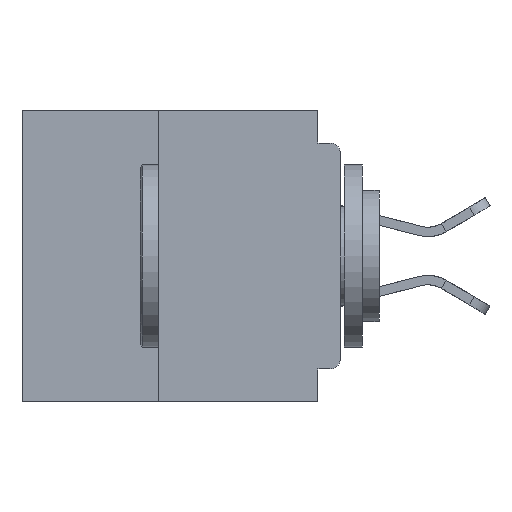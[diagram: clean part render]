
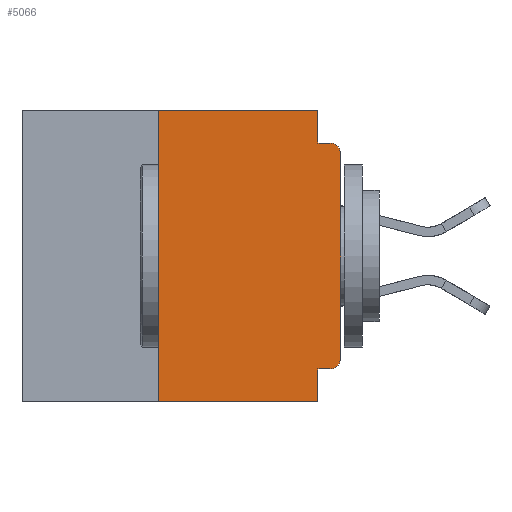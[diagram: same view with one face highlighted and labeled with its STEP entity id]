
A CAD part, left-side view. The second image highlights one B-rep face of the part: STEP entity #5066.
In plain terms, the highlighted planar face has unit normal (-1, 0, 0).
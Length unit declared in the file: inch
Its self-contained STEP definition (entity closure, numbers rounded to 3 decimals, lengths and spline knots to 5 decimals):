
#410 = VERTEX_POINT ( 'NONE', #44594 ) ;
#521 = CARTESIAN_POINT ( 'NONE',  ( 0., 0.015, -0.045 ) ) ;
#858 = CARTESIAN_POINT ( 'NONE',  ( 0., 0.25, -0.4 ) ) ;
#1553 = VERTEX_POINT ( 'NONE', #38633 ) ;
#1782 = EDGE_CURVE ( 'NONE', #38495, #410, #31186, .T. ) ;
#2351 = VECTOR ( 'NONE', #15115, 39.37008 ) ;
#2482 = LINE ( 'NONE', #26480, #40774 ) ;
#2640 = DIRECTION ( 'NONE',  ( 0., 0., -1. ) ) ;
#2669 = DIRECTION ( 'NONE',  ( 0., 0., -1. ) ) ;
#3122 = DIRECTION ( 'NONE',  ( 0., -1., 0. ) ) ;
#3851 = EDGE_CURVE ( 'NONE', #36804, #38495, #11431, .T. ) ;
#5031 = VECTOR ( 'NONE', #39008, 39.37008 ) ;
#5066 = ADVANCED_FACE ( 'NONE', ( #44880 ), #32193, .F. ) ;
#5093 = EDGE_CURVE ( 'NONE', #30592, #1553, #25356, .T. ) ;
#5676 = AXIS2_PLACEMENT_3D ( 'NONE', #14829, #40547, #18569 ) ;
#6578 = ORIENTED_EDGE ( 'NONE', *, *, #15132, .T. ) ;
#6948 = EDGE_CURVE ( 'NONE', #1553, #24977, #2482, .T. ) ;
#7281 = VERTEX_POINT ( 'NONE', #17346 ) ;
#7974 = CARTESIAN_POINT ( 'NONE',  ( 0., 0.031, 0. ) ) ;
#8047 = EDGE_CURVE ( 'NONE', #7281, #14858, #14187, .T. ) ;
#8215 = ORIENTED_EDGE ( 'NONE', *, *, #16314, .F. ) ;
#8944 = CARTESIAN_POINT ( 'NONE',  ( 0., 0.031, -0.355 ) ) ;
#9020 = DIRECTION ( 'NONE',  ( 0., 0., -1. ) ) ;
#9783 = AXIS2_PLACEMENT_3D ( 'NONE', #21483, #47158, #25150 ) ;
#10757 = CARTESIAN_POINT ( 'NONE',  ( 0., 0.031, 0. ) ) ;
#11431 = LINE ( 'NONE', #32276, #20201 ) ;
#12268 = DIRECTION ( 'NONE',  ( 0., 0., 1. ) ) ;
#12294 = AXIS2_PLACEMENT_3D ( 'NONE', #46854, #24986, #2640 ) ;
#12662 = LINE ( 'NONE', #28679, #29947 ) ;
#14187 = LINE ( 'NONE', #18089, #21715 ) ;
#14800 = VERTEX_POINT ( 'NONE', #8944 ) ;
#14829 = CARTESIAN_POINT ( 'NONE',  ( 0., 0.015, -0.06 ) ) ;
#14858 = VERTEX_POINT ( 'NONE', #31234 ) ;
#15036 = LINE ( 'NONE', #42671, #5031 ) ;
#15115 = DIRECTION ( 'NONE',  ( 0., -1., 0. ) ) ;
#15132 = EDGE_CURVE ( 'NONE', #24977, #17770, #23715, .T. ) ;
#16197 = EDGE_CURVE ( 'NONE', #30592, #14800, #15036, .T. ) ;
#16314 = EDGE_CURVE ( 'NONE', #14800, #14858, #12662, .T. ) ;
#17346 = CARTESIAN_POINT ( 'NONE',  ( 0., 0.25, -0.4 ) ) ;
#17770 = VERTEX_POINT ( 'NONE', #521 ) ;
#18029 = EDGE_LOOP ( 'NONE', ( #35702, #6578, #40724, #28450, #26901, #32631, #36878, #8215, #34798, #23837 ) ) ;
#18089 = CARTESIAN_POINT ( 'NONE',  ( 0., 0.437, -0.4 ) ) ;
#18569 = DIRECTION ( 'NONE',  ( 0., 0., -1. ) ) ;
#20201 = VECTOR ( 'NONE', #46948, 39.37008 ) ;
#21483 = CARTESIAN_POINT ( 'NONE',  ( 0., 0.015, -0.34 ) ) ;
#21715 = VECTOR ( 'NONE', #3122, 39.37008 ) ;
#23715 = CIRCLE ( 'NONE', #5676, 0.015 ) ;
#23837 = ORIENTED_EDGE ( 'NONE', *, *, #5093, .T. ) ;
#24977 = VERTEX_POINT ( 'NONE', #38444 ) ;
#24986 = DIRECTION ( 'NONE',  ( 1., 0., 0. ) ) ;
#25150 = DIRECTION ( 'NONE',  ( 0., 0., -1. ) ) ;
#25345 = EDGE_CURVE ( 'NONE', #410, #17770, #28521, .T. ) ;
#25356 = CIRCLE ( 'NONE', #9783, 0.015 ) ;
#25401 = VECTOR ( 'NONE', #12268, 39.37008 ) ;
#25553 = CARTESIAN_POINT ( 'NONE',  ( 0., 0.015, -0.355 ) ) ;
#26480 = CARTESIAN_POINT ( 'NONE',  ( 0., 0., 0. ) ) ;
#26901 = ORIENTED_EDGE ( 'NONE', *, *, #3851, .F. ) ;
#28450 = ORIENTED_EDGE ( 'NONE', *, *, #1782, .F. ) ;
#28521 = LINE ( 'NONE', #37136, #2351 ) ;
#28679 = CARTESIAN_POINT ( 'NONE',  ( 0., 0.031, -0.4 ) ) ;
#29947 = VECTOR ( 'NONE', #2669, 39.37008 ) ;
#30592 = VERTEX_POINT ( 'NONE', #25553 ) ;
#31186 = LINE ( 'NONE', #10757, #39849 ) ;
#31234 = CARTESIAN_POINT ( 'NONE',  ( 0., 0.031, -0.4 ) ) ;
#32193 = PLANE ( 'NONE',  #12294 ) ;
#32276 = CARTESIAN_POINT ( 'NONE',  ( 0., 0.437, 0. ) ) ;
#32631 = ORIENTED_EDGE ( 'NONE', *, *, #37992, .F. ) ;
#34472 = CARTESIAN_POINT ( 'NONE',  ( 0., 0.25, 0. ) ) ;
#34798 = ORIENTED_EDGE ( 'NONE', *, *, #16197, .F. ) ;
#35155 = LINE ( 'NONE', #858, #25401 ) ;
#35702 = ORIENTED_EDGE ( 'NONE', *, *, #6948, .T. ) ;
#36804 = VERTEX_POINT ( 'NONE', #34472 ) ;
#36878 = ORIENTED_EDGE ( 'NONE', *, *, #8047, .T. ) ;
#37136 = CARTESIAN_POINT ( 'NONE',  ( 0., 0., -0.045 ) ) ;
#37582 = DIRECTION ( 'NONE',  ( 0., 0., 1. ) ) ;
#37992 = EDGE_CURVE ( 'NONE', #7281, #36804, #35155, .T. ) ;
#38444 = CARTESIAN_POINT ( 'NONE',  ( 0., 0., -0.06 ) ) ;
#38495 = VERTEX_POINT ( 'NONE', #7974 ) ;
#38633 = CARTESIAN_POINT ( 'NONE',  ( 0., 0., -0.34 ) ) ;
#39008 = DIRECTION ( 'NONE',  ( 0., 1., 0. ) ) ;
#39849 = VECTOR ( 'NONE', #9020, 39.37008 ) ;
#40547 = DIRECTION ( 'NONE',  ( -1., 0., 0. ) ) ;
#40724 = ORIENTED_EDGE ( 'NONE', *, *, #25345, .F. ) ;
#40774 = VECTOR ( 'NONE', #37582, 39.37008 ) ;
#42671 = CARTESIAN_POINT ( 'NONE',  ( 0., 0., -0.355 ) ) ;
#44594 = CARTESIAN_POINT ( 'NONE',  ( 0., 0.031, -0.045 ) ) ;
#44880 = FACE_OUTER_BOUND ( 'NONE', #18029, .T. ) ;
#46854 = CARTESIAN_POINT ( 'NONE',  ( 0., 0.437, 0. ) ) ;
#46948 = DIRECTION ( 'NONE',  ( 0., -1., 0. ) ) ;
#47158 = DIRECTION ( 'NONE',  ( -1., 0., 0. ) ) ;
